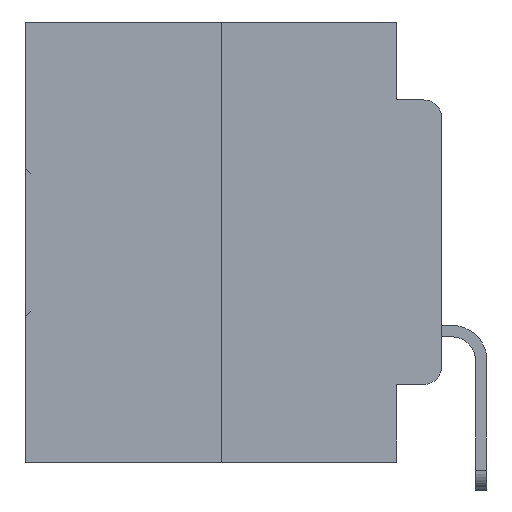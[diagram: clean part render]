
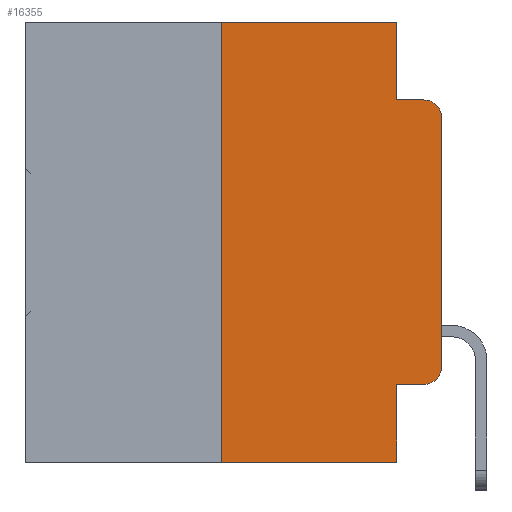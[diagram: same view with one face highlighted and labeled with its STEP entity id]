
A CAD part, left-side view. The second image highlights one B-rep face of the part: STEP entity #16355.
In plain terms, the highlighted planar face has unit normal (-1, 0, 0).
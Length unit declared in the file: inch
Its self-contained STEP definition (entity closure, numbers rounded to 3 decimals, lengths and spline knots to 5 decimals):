
#176 = CARTESIAN_POINT ( 'NONE',  ( 0., 0.473, -0.5 ) ) ;
#454 = DIRECTION ( 'NONE',  ( 0., 0., 1. ) ) ;
#729 = LINE ( 'NONE', #12108, #14591 ) ;
#942 = ORIENTED_EDGE ( 'NONE', *, *, #1573, .F. ) ;
#1234 = VERTEX_POINT ( 'NONE', #25943 ) ;
#1454 = VECTOR ( 'NONE', #26349, 39.37008 ) ;
#1573 = EDGE_CURVE ( 'NONE', #9039, #6460, #9353, .T. ) ;
#2002 = CARTESIAN_POINT ( 'NONE',  ( 0., 0.051, -0.4115 ) ) ;
#2888 = DIRECTION ( 'NONE',  ( 0., -1., 0. ) ) ;
#3290 = ORIENTED_EDGE ( 'NONE', *, *, #8742, .F. ) ;
#3551 = LINE ( 'NONE', #23654, #17225 ) ;
#4279 = DIRECTION ( 'NONE',  ( 0., 0., -1. ) ) ;
#4709 = VERTEX_POINT ( 'NONE', #24080 ) ;
#5122 = ORIENTED_EDGE ( 'NONE', *, *, #12098, .T. ) ;
#5154 = VERTEX_POINT ( 'NONE', #6841 ) ;
#5427 = DIRECTION ( 'NONE',  ( -1., 0., 0. ) ) ;
#5832 = DIRECTION ( 'NONE',  ( 0., 0., -1. ) ) ;
#6414 = CARTESIAN_POINT ( 'NONE',  ( 0., 0., -0.3915 ) ) ;
#6460 = VERTEX_POINT ( 'NONE', #12490 ) ;
#6486 = VERTEX_POINT ( 'NONE', #7611 ) ;
#6841 = CARTESIAN_POINT ( 'NONE',  ( 0., 0.02, -0.0885 ) ) ;
#7611 = CARTESIAN_POINT ( 'NONE',  ( 0., 0.051, -0.5 ) ) ;
#8525 = EDGE_CURVE ( 'NONE', #9039, #6486, #10203, .T. ) ;
#8625 = AXIS2_PLACEMENT_3D ( 'NONE', #20528, #5427, #22891 ) ;
#8728 = VERTEX_POINT ( 'NONE', #21274 ) ;
#8742 = EDGE_CURVE ( 'NONE', #4709, #27760, #3551, .T. ) ;
#8753 = VERTEX_POINT ( 'NONE', #6414 ) ;
#8829 = DIRECTION ( 'NONE',  ( -1., 0., 0. ) ) ;
#9039 = VERTEX_POINT ( 'NONE', #17580 ) ;
#9082 = VECTOR ( 'NONE', #17542, 39.37008 ) ;
#9353 = LINE ( 'NONE', #28734, #1454 ) ;
#10203 = LINE ( 'NONE', #176, #16088 ) ;
#10439 = EDGE_CURVE ( 'NONE', #27760, #5154, #729, .T. ) ;
#10870 = AXIS2_PLACEMENT_3D ( 'NONE', #25532, #20870, #5832 ) ;
#11499 = DIRECTION ( 'NONE',  ( 0., 0., -1. ) ) ;
#11543 = VECTOR ( 'NONE', #4279, 39.37008 ) ;
#11586 = ORIENTED_EDGE ( 'NONE', *, *, #23190, .F. ) ;
#12019 = FACE_OUTER_BOUND ( 'NONE', #18891, .T. ) ;
#12098 = EDGE_CURVE ( 'NONE', #8728, #5154, #31731, .T. ) ;
#12108 = CARTESIAN_POINT ( 'NONE',  ( 0., 0.051, -0.0885 ) ) ;
#12175 = CARTESIAN_POINT ( 'NONE',  ( 0., 0.051, -0.0885 ) ) ;
#12490 = CARTESIAN_POINT ( 'NONE',  ( 0., 0.25, 0. ) ) ;
#13787 = VERTEX_POINT ( 'NONE', #17648 ) ;
#13802 = ORIENTED_EDGE ( 'NONE', *, *, #25751, .T. ) ;
#14018 = ORIENTED_EDGE ( 'NONE', *, *, #21957, .T. ) ;
#14591 = VECTOR ( 'NONE', #14664, 39.37008 ) ;
#14664 = DIRECTION ( 'NONE',  ( 0., -1., 0. ) ) ;
#15142 = CARTESIAN_POINT ( 'NONE',  ( 0., 0.473, 0. ) ) ;
#16088 = VECTOR ( 'NONE', #2888, 39.37008 ) ;
#16277 = LINE ( 'NONE', #15142, #21179 ) ;
#16355 = ADVANCED_FACE ( 'NONE', ( #12019 ), #18466, .F. ) ;
#17225 = VECTOR ( 'NONE', #11499, 39.37008 ) ;
#17542 = DIRECTION ( 'NONE',  ( 0., -1., 0. ) ) ;
#17580 = CARTESIAN_POINT ( 'NONE',  ( 0., 0.25, -0.5 ) ) ;
#17648 = CARTESIAN_POINT ( 'NONE',  ( 0., 0.051, -0.4115 ) ) ;
#18466 = PLANE ( 'NONE',  #10870 ) ;
#18519 = ORIENTED_EDGE ( 'NONE', *, *, #10439, .F. ) ;
#18891 = EDGE_LOOP ( 'NONE', ( #14018, #5122, #18519, #3290, #11586, #942, #29109, #29439, #13802, #30979 ) ) ;
#20127 = LINE ( 'NONE', #30336, #25700 ) ;
#20528 = CARTESIAN_POINT ( 'NONE',  ( 0., 0.02, -0.3915 ) ) ;
#20870 = DIRECTION ( 'NONE',  ( 1., 0., 0. ) ) ;
#21179 = VECTOR ( 'NONE', #27089, 39.37008 ) ;
#21274 = CARTESIAN_POINT ( 'NONE',  ( 0., 0., -0.1085 ) ) ;
#21957 = EDGE_CURVE ( 'NONE', #8753, #8728, #20127, .T. ) ;
#22175 = LINE ( 'NONE', #2002, #9082 ) ;
#22891 = DIRECTION ( 'NONE',  ( 0., 0., -1. ) ) ;
#23190 = EDGE_CURVE ( 'NONE', #6460, #4709, #16277, .T. ) ;
#23542 = CARTESIAN_POINT ( 'NONE',  ( 0., 0.02, -0.1085 ) ) ;
#23654 = CARTESIAN_POINT ( 'NONE',  ( 0., 0.051, 0. ) ) ;
#24080 = CARTESIAN_POINT ( 'NONE',  ( 0., 0.051, 0. ) ) ;
#24154 = EDGE_CURVE ( 'NONE', #1234, #8753, #28934, .T. ) ;
#24493 = LINE ( 'NONE', #26677, #11543 ) ;
#24875 = AXIS2_PLACEMENT_3D ( 'NONE', #23542, #8829, #25944 ) ;
#25532 = CARTESIAN_POINT ( 'NONE',  ( 0., 0.473, 0. ) ) ;
#25700 = VECTOR ( 'NONE', #454, 39.37008 ) ;
#25751 = EDGE_CURVE ( 'NONE', #13787, #1234, #22175, .T. ) ;
#25943 = CARTESIAN_POINT ( 'NONE',  ( 0., 0.02, -0.4115 ) ) ;
#25944 = DIRECTION ( 'NONE',  ( 0., 0., -1. ) ) ;
#26349 = DIRECTION ( 'NONE',  ( 0., 0., 1. ) ) ;
#26677 = CARTESIAN_POINT ( 'NONE',  ( 0., 0.051, 0. ) ) ;
#27089 = DIRECTION ( 'NONE',  ( 0., -1., 0. ) ) ;
#27760 = VERTEX_POINT ( 'NONE', #12175 ) ;
#28734 = CARTESIAN_POINT ( 'NONE',  ( 0., 0.25, 0. ) ) ;
#28934 = CIRCLE ( 'NONE', #8625, 0.02 ) ;
#29109 = ORIENTED_EDGE ( 'NONE', *, *, #8525, .T. ) ;
#29439 = ORIENTED_EDGE ( 'NONE', *, *, #32128, .F. ) ;
#30336 = CARTESIAN_POINT ( 'NONE',  ( 0., 0., 0. ) ) ;
#30979 = ORIENTED_EDGE ( 'NONE', *, *, #24154, .T. ) ;
#31731 = CIRCLE ( 'NONE', #24875, 0.02 ) ;
#32128 = EDGE_CURVE ( 'NONE', #13787, #6486, #24493, .T. ) ;
